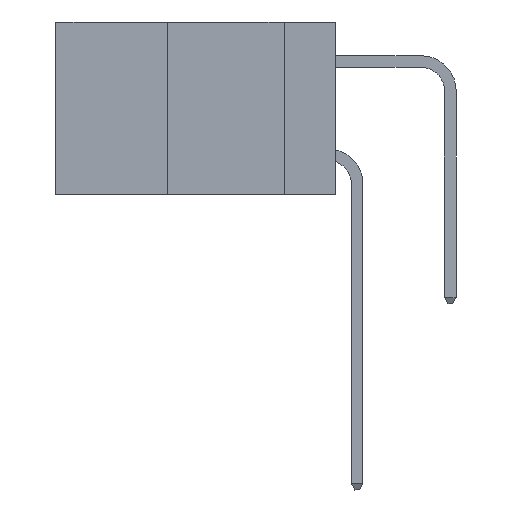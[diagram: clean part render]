
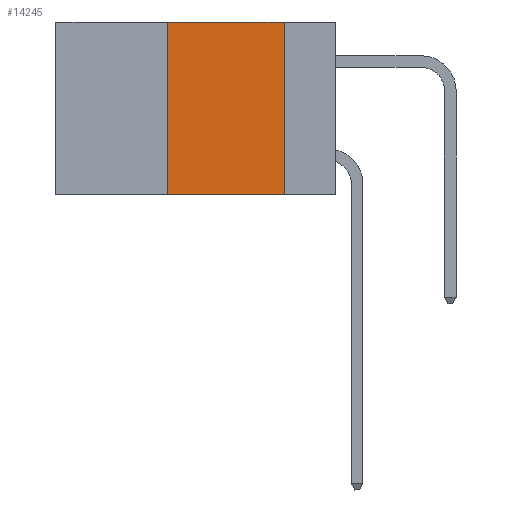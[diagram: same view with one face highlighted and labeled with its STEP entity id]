
A CAD part, left-side view. The second image highlights one B-rep face of the part: STEP entity #14245.
In plain terms, the highlighted planar face has unit normal (-1, 0, 0).
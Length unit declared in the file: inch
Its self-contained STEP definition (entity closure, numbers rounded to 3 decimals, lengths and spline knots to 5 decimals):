
#128 = EDGE_CURVE ( 'NONE', #8796, #6777, #9042, .T. ) ;
#609 = DIRECTION ( 'NONE',  ( 0., 0., 1. ) ) ;
#1459 = VERTEX_POINT ( 'NONE', #17648 ) ;
#1754 = LINE ( 'NONE', #22434, #3282 ) ;
#2068 = ORIENTED_EDGE ( 'NONE', *, *, #22848, .F. ) ;
#2752 = DIRECTION ( 'NONE',  ( 1., 0., 0. ) ) ;
#2949 = CARTESIAN_POINT ( 'NONE',  ( 0., 0.11, -0.37 ) ) ;
#3282 = VECTOR ( 'NONE', #10517, 39.37008 ) ;
#3915 = LINE ( 'NONE', #11834, #5768 ) ;
#4311 = DIRECTION ( 'NONE',  ( 0., -1., 0. ) ) ;
#4484 = VECTOR ( 'NONE', #5356, 39.37008 ) ;
#5356 = DIRECTION ( 'NONE',  ( 0., 0., -1. ) ) ;
#5768 = VECTOR ( 'NONE', #609, 39.37008 ) ;
#6147 = EDGE_CURVE ( 'NONE', #8395, #1459, #1754, .T. ) ;
#6777 = VERTEX_POINT ( 'NONE', #2949 ) ;
#8395 = VERTEX_POINT ( 'NONE', #22249 ) ;
#8796 = VERTEX_POINT ( 'NONE', #24940 ) ;
#9042 = LINE ( 'NONE', #23738, #9968 ) ;
#9968 = VECTOR ( 'NONE', #4311, 39.37008 ) ;
#10517 = DIRECTION ( 'NONE',  ( 0., -1., 0. ) ) ;
#10807 = DIRECTION ( 'NONE',  ( 0., 0., -1. ) ) ;
#11834 = CARTESIAN_POINT ( 'NONE',  ( 0., 0.36, 0. ) ) ;
#12503 = LINE ( 'NONE', #19414, #4484 ) ;
#13738 = ORIENTED_EDGE ( 'NONE', *, *, #6147, .F. ) ;
#14245 = ADVANCED_FACE ( 'NONE', ( #19936 ), #22789, .F. ) ;
#16635 = CARTESIAN_POINT ( 'NONE',  ( 0., 0.6, 0. ) ) ;
#17433 = ORIENTED_EDGE ( 'NONE', *, *, #128, .T. ) ;
#17648 = CARTESIAN_POINT ( 'NONE',  ( 0., 0.11, 0. ) ) ;
#18094 = EDGE_LOOP ( 'NONE', ( #20588, #13738, #2068, #17433 ) ) ;
#19414 = CARTESIAN_POINT ( 'NONE',  ( 0., 0.11, 0. ) ) ;
#19936 = FACE_OUTER_BOUND ( 'NONE', #18094, .T. ) ;
#20588 = ORIENTED_EDGE ( 'NONE', *, *, #23799, .F. ) ;
#22249 = CARTESIAN_POINT ( 'NONE',  ( 0., 0.36, 0. ) ) ;
#22434 = CARTESIAN_POINT ( 'NONE',  ( 0., 0.6, 0. ) ) ;
#22789 = PLANE ( 'NONE',  #24079 ) ;
#22848 = EDGE_CURVE ( 'NONE', #8796, #8395, #3915, .T. ) ;
#23738 = CARTESIAN_POINT ( 'NONE',  ( 0., 0.6, -0.37 ) ) ;
#23799 = EDGE_CURVE ( 'NONE', #1459, #6777, #12503, .T. ) ;
#24079 = AXIS2_PLACEMENT_3D ( 'NONE', #16635, #2752, #10807 ) ;
#24940 = CARTESIAN_POINT ( 'NONE',  ( 0., 0.36, -0.37 ) ) ;
